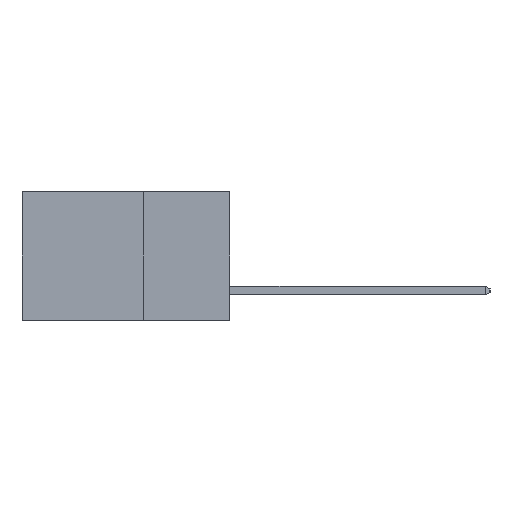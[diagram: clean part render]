
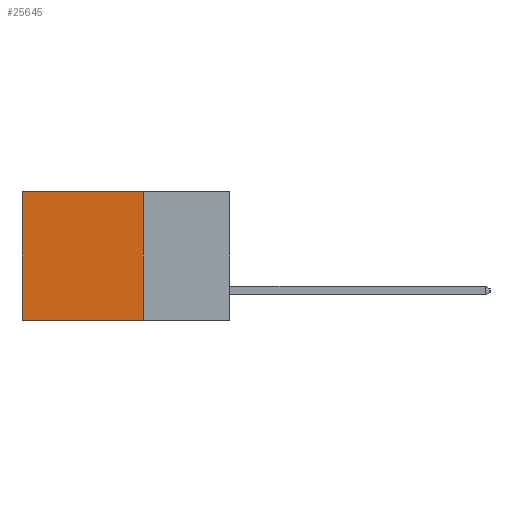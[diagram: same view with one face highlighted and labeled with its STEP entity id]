
A CAD part, left-side view. The second image highlights one B-rep face of the part: STEP entity #25645.
In plain terms, the highlighted planar face has unit normal (-1, 0, 0).
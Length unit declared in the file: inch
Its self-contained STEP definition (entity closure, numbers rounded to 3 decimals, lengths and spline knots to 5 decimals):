
#529 = CARTESIAN_POINT ( 'NONE',  ( 0.298, 0.25, 0. ) ) ;
#1099 = DIRECTION ( 'NONE',  ( 0., 1., 0. ) ) ;
#1167 = CARTESIAN_POINT ( 'NONE',  ( 0.298, 0.25, 0. ) ) ;
#2401 = FACE_OUTER_BOUND ( 'NONE', #13466, .T. ) ;
#3641 = LINE ( 'NONE', #1167, #27397 ) ;
#4631 = CARTESIAN_POINT ( 'NONE',  ( 0.298, 0.25, -0.37 ) ) ;
#5128 = DIRECTION ( 'NONE',  ( 0., 0., -1. ) ) ;
#6100 = CARTESIAN_POINT ( 'NONE',  ( 0.298, 0.6, -0.37 ) ) ;
#7375 = EDGE_CURVE ( 'NONE', #14892, #25310, #3641, .T. ) ;
#8412 = CARTESIAN_POINT ( 'NONE',  ( 0.298, 0.25, 0. ) ) ;
#10712 = ORIENTED_EDGE ( 'NONE', *, *, #7375, .T. ) ;
#11462 = VECTOR ( 'NONE', #23367, 39.37008 ) ;
#12204 = VECTOR ( 'NONE', #28820, 39.37008 ) ;
#12697 = ORIENTED_EDGE ( 'NONE', *, *, #27032, .F. ) ;
#12707 = LINE ( 'NONE', #18530, #24225 ) ;
#13466 = EDGE_LOOP ( 'NONE', ( #26030, #12697, #24682, #10712 ) ) ;
#13658 = CARTESIAN_POINT ( 'NONE',  ( 0.298, 0.6, 0. ) ) ;
#14892 = VERTEX_POINT ( 'NONE', #8412 ) ;
#16413 = CARTESIAN_POINT ( 'NONE',  ( 0.298, 0.25, 0. ) ) ;
#16625 = PLANE ( 'NONE',  #21458 ) ;
#17578 = LINE ( 'NONE', #16413, #11462 ) ;
#18530 = CARTESIAN_POINT ( 'NONE',  ( 0.298, 0.6, 0. ) ) ;
#18929 = DIRECTION ( 'NONE',  ( 1., 0., 0. ) ) ;
#19652 = VERTEX_POINT ( 'NONE', #4631 ) ;
#20807 = DIRECTION ( 'NONE',  ( 0., 0., -1. ) ) ;
#21458 = AXIS2_PLACEMENT_3D ( 'NONE', #529, #18929, #5128 ) ;
#21659 = EDGE_CURVE ( 'NONE', #25310, #22025, #12707, .T. ) ;
#22025 = VERTEX_POINT ( 'NONE', #6100 ) ;
#23367 = DIRECTION ( 'NONE',  ( 0., 0., -1. ) ) ;
#24225 = VECTOR ( 'NONE', #20807, 39.37008 ) ;
#24466 = LINE ( 'NONE', #26511, #12204 ) ;
#24682 = ORIENTED_EDGE ( 'NONE', *, *, #27462, .F. ) ;
#25310 = VERTEX_POINT ( 'NONE', #13658 ) ;
#25645 = ADVANCED_FACE ( 'NONE', ( #2401 ), #16625, .F. ) ;
#26030 = ORIENTED_EDGE ( 'NONE', *, *, #21659, .T. ) ;
#26511 = CARTESIAN_POINT ( 'NONE',  ( 0.298, 0.25, -0.37 ) ) ;
#27032 = EDGE_CURVE ( 'NONE', #19652, #22025, #24466, .T. ) ;
#27397 = VECTOR ( 'NONE', #1099, 39.37008 ) ;
#27462 = EDGE_CURVE ( 'NONE', #14892, #19652, #17578, .T. ) ;
#28820 = DIRECTION ( 'NONE',  ( 0., 1., 0. ) ) ;
